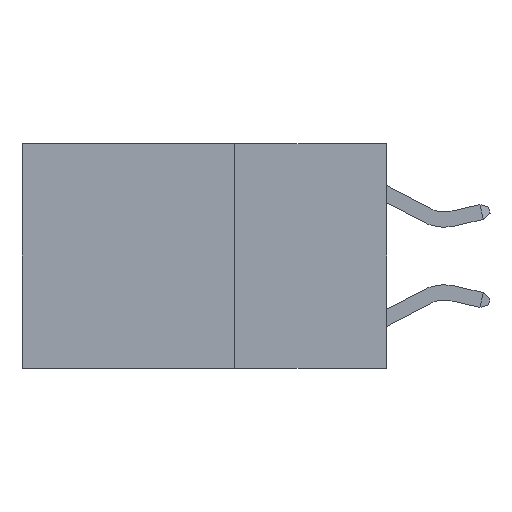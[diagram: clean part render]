
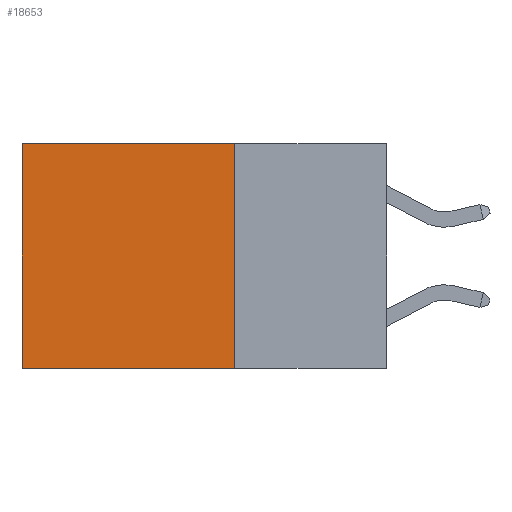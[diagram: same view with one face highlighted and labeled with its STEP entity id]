
A CAD part, left-side view. The second image highlights one B-rep face of the part: STEP entity #18653.
In plain terms, the highlighted planar face has unit normal (-1, 0, 0).
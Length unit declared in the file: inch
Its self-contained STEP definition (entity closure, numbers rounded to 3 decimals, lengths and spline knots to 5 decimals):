
#509 = VECTOR ( 'NONE', #16747, 39.37008 ) ;
#1802 = EDGE_LOOP ( 'NONE', ( #29754, #13184, #19672, #13222 ) ) ;
#2595 = CARTESIAN_POINT ( 'NONE',  ( 0.2625, 0.25, -0.37 ) ) ;
#3353 = CARTESIAN_POINT ( 'NONE',  ( 0.2625, 0.25, 0. ) ) ;
#3507 = DIRECTION ( 'NONE',  ( 0., 1., 0. ) ) ;
#3832 = CARTESIAN_POINT ( 'NONE',  ( 0.2625, 0.6, 0. ) ) ;
#4112 = DIRECTION ( 'NONE',  ( 0., 1., 0. ) ) ;
#6501 = LINE ( 'NONE', #20685, #26889 ) ;
#6531 = VERTEX_POINT ( 'NONE', #2595 ) ;
#6927 = EDGE_CURVE ( 'NONE', #18600, #6531, #6501, .T. ) ;
#7073 = AXIS2_PLACEMENT_3D ( 'NONE', #15321, #22493, #22178 ) ;
#7202 = CARTESIAN_POINT ( 'NONE',  ( 0.2625, 0.6, 0. ) ) ;
#8435 = LINE ( 'NONE', #3353, #20883 ) ;
#11109 = LINE ( 'NONE', #20825, #17159 ) ;
#11416 = EDGE_CURVE ( 'NONE', #18600, #18934, #8435, .T. ) ;
#12467 = PLANE ( 'NONE',  #7073 ) ;
#13184 = ORIENTED_EDGE ( 'NONE', *, *, #29271, .F. ) ;
#13222 = ORIENTED_EDGE ( 'NONE', *, *, #11416, .T. ) ;
#15321 = CARTESIAN_POINT ( 'NONE',  ( 0.2625, 0.25, 0. ) ) ;
#15534 = EDGE_CURVE ( 'NONE', #18934, #25702, #18645, .T. ) ;
#16747 = DIRECTION ( 'NONE',  ( 0., 0., -1. ) ) ;
#17159 = VECTOR ( 'NONE', #4112, 39.37008 ) ;
#18600 = VERTEX_POINT ( 'NONE', #26960 ) ;
#18645 = LINE ( 'NONE', #7202, #509 ) ;
#18653 = ADVANCED_FACE ( 'NONE', ( #24702 ), #12467, .F. ) ;
#18934 = VERTEX_POINT ( 'NONE', #3832 ) ;
#19672 = ORIENTED_EDGE ( 'NONE', *, *, #6927, .F. ) ;
#20685 = CARTESIAN_POINT ( 'NONE',  ( 0.2625, 0.25, 0. ) ) ;
#20825 = CARTESIAN_POINT ( 'NONE',  ( 0.2625, 0.25, -0.37 ) ) ;
#20883 = VECTOR ( 'NONE', #3507, 39.37008 ) ;
#22178 = DIRECTION ( 'NONE',  ( 0., 0., -1. ) ) ;
#22493 = DIRECTION ( 'NONE',  ( 1., 0., 0. ) ) ;
#24702 = FACE_OUTER_BOUND ( 'NONE', #1802, .T. ) ;
#25702 = VERTEX_POINT ( 'NONE', #30812 ) ;
#26889 = VECTOR ( 'NONE', #30575, 39.37008 ) ;
#26960 = CARTESIAN_POINT ( 'NONE',  ( 0.2625, 0.25, 0. ) ) ;
#29271 = EDGE_CURVE ( 'NONE', #6531, #25702, #11109, .T. ) ;
#29754 = ORIENTED_EDGE ( 'NONE', *, *, #15534, .T. ) ;
#30575 = DIRECTION ( 'NONE',  ( 0., 0., -1. ) ) ;
#30812 = CARTESIAN_POINT ( 'NONE',  ( 0.2625, 0.6, -0.37 ) ) ;
